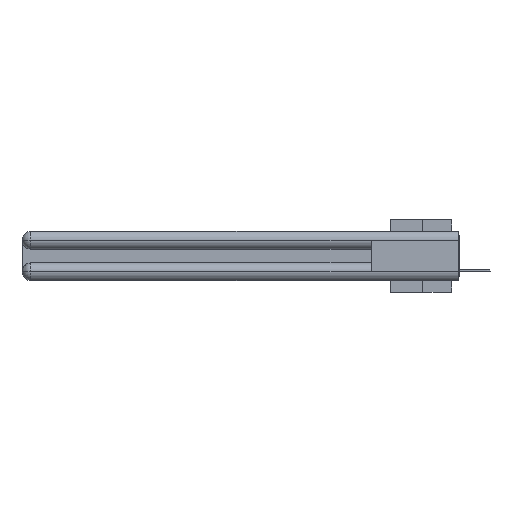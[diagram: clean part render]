
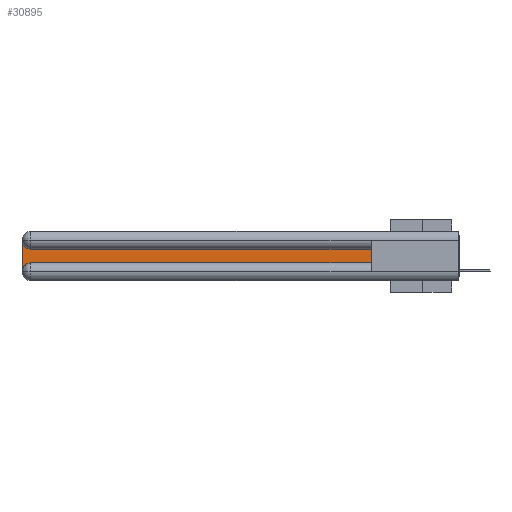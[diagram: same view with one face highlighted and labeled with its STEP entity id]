
A CAD part, left-side view. The second image highlights one B-rep face of the part: STEP entity #30895.
In plain terms, the highlighted planar face has unit normal (-1, 0, 0).
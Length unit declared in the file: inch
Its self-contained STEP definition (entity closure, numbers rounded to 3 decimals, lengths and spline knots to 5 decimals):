
#34 = VECTOR ( 'NONE', #32106, 39.37008 ) ;
#183 = FACE_OUTER_BOUND ( 'NONE', #7067, .T. ) ;
#458 = DIRECTION ( 'NONE',  ( 0., 0., 1. ) ) ;
#1722 = CARTESIAN_POINT ( 'NONE',  ( 0.075, 3., -0.2775 ) ) ;
#2449 = ORIENTED_EDGE ( 'NONE', *, *, #33155, .T. ) ;
#3224 = VECTOR ( 'NONE', #24796, 39.37008 ) ;
#3595 = DIRECTION ( 'NONE',  ( 1., 0., 0. ) ) ;
#3738 = CARTESIAN_POINT ( 'NONE',  ( 0.075, 0.6, -0.2175 ) ) ;
#3986 = VERTEX_POINT ( 'NONE', #9691 ) ;
#4912 = ORIENTED_EDGE ( 'NONE', *, *, #9666, .T. ) ;
#5018 = DIRECTION ( 'NONE',  ( 0., 0., -1. ) ) ;
#5231 = CARTESIAN_POINT ( 'NONE',  ( 0.075, 0.6, -0.1225 ) ) ;
#5676 = VERTEX_POINT ( 'NONE', #24469 ) ;
#6238 = AXIS2_PLACEMENT_3D ( 'NONE', #24246, #32533, #21610 ) ;
#6283 = VECTOR ( 'NONE', #5018, 39.37008 ) ;
#6304 = CARTESIAN_POINT ( 'NONE',  ( 0.075, 0.6, -0.2175 ) ) ;
#7067 = EDGE_LOOP ( 'NONE', ( #29985, #26607, #31412, #24740, #2449, #4912 ) ) ;
#7433 = EDGE_CURVE ( 'NONE', #22958, #35300, #23633, .T. ) ;
#7541 = EDGE_CURVE ( 'NONE', #20735, #34214, #7695, .T. ) ;
#7695 = LINE ( 'NONE', #5231, #3224 ) ;
#8851 = DIRECTION ( 'NONE',  ( 0., 0., -1. ) ) ;
#9108 = CIRCLE ( 'NONE', #18108, 0.06 ) ;
#9666 = EDGE_CURVE ( 'NONE', #5676, #20735, #26212, .T. ) ;
#9691 = CARTESIAN_POINT ( 'NONE',  ( 0.075, 3., -0.0625 ) ) ;
#15067 = DIRECTION ( 'NONE',  ( 0., 0., -1. ) ) ;
#16192 = AXIS2_PLACEMENT_3D ( 'NONE', #28204, #28559, #8851 ) ;
#16713 = CARTESIAN_POINT ( 'NONE',  ( 0.075, 2.94, -0.1225 ) ) ;
#18108 = AXIS2_PLACEMENT_3D ( 'NONE', #29126, #3595, #15067 ) ;
#20627 = LINE ( 'NONE', #3738, #34 ) ;
#20735 = VERTEX_POINT ( 'NONE', #32640 ) ;
#21610 = DIRECTION ( 'NONE',  ( 0., 0., -1. ) ) ;
#22958 = VERTEX_POINT ( 'NONE', #1722 ) ;
#23633 = CIRCLE ( 'NONE', #6238, 0.06 ) ;
#24246 = CARTESIAN_POINT ( 'NONE',  ( 0.075, 2.94, -0.2775 ) ) ;
#24469 = CARTESIAN_POINT ( 'NONE',  ( 0.075, 0.6, -0.2175 ) ) ;
#24581 = LINE ( 'NONE', #24926, #6283 ) ;
#24740 = ORIENTED_EDGE ( 'NONE', *, *, #7433, .T. ) ;
#24796 = DIRECTION ( 'NONE',  ( 0., 1., 0. ) ) ;
#24926 = CARTESIAN_POINT ( 'NONE',  ( 0.075, 3., -0.2175 ) ) ;
#25953 = PLANE ( 'NONE',  #16192 ) ;
#26212 = LINE ( 'NONE', #6304, #33956 ) ;
#26607 = ORIENTED_EDGE ( 'NONE', *, *, #32714, .T. ) ;
#28204 = CARTESIAN_POINT ( 'NONE',  ( 0.075, 3., -0.1225 ) ) ;
#28559 = DIRECTION ( 'NONE',  ( 1., 0., 0. ) ) ;
#29126 = CARTESIAN_POINT ( 'NONE',  ( 0.075, 2.94, -0.0625 ) ) ;
#29985 = ORIENTED_EDGE ( 'NONE', *, *, #7541, .T. ) ;
#30094 = CARTESIAN_POINT ( 'NONE',  ( 0.075, 2.94, -0.2175 ) ) ;
#30895 = ADVANCED_FACE ( 'NONE', ( #183 ), #25953, .F. ) ;
#31412 = ORIENTED_EDGE ( 'NONE', *, *, #36390, .T. ) ;
#32106 = DIRECTION ( 'NONE',  ( 0., -1., 0. ) ) ;
#32533 = DIRECTION ( 'NONE',  ( 1., 0., 0. ) ) ;
#32640 = CARTESIAN_POINT ( 'NONE',  ( 0.075, 0.6, -0.1225 ) ) ;
#32714 = EDGE_CURVE ( 'NONE', #34214, #3986, #9108, .T. ) ;
#33155 = EDGE_CURVE ( 'NONE', #35300, #5676, #20627, .T. ) ;
#33956 = VECTOR ( 'NONE', #458, 39.37008 ) ;
#34214 = VERTEX_POINT ( 'NONE', #16713 ) ;
#35300 = VERTEX_POINT ( 'NONE', #30094 ) ;
#36390 = EDGE_CURVE ( 'NONE', #3986, #22958, #24581, .T. ) ;
